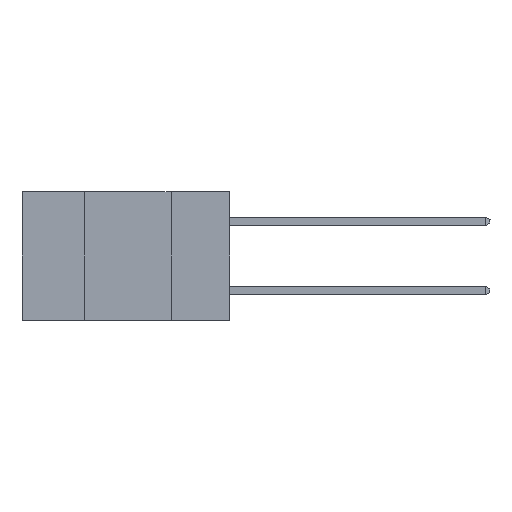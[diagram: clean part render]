
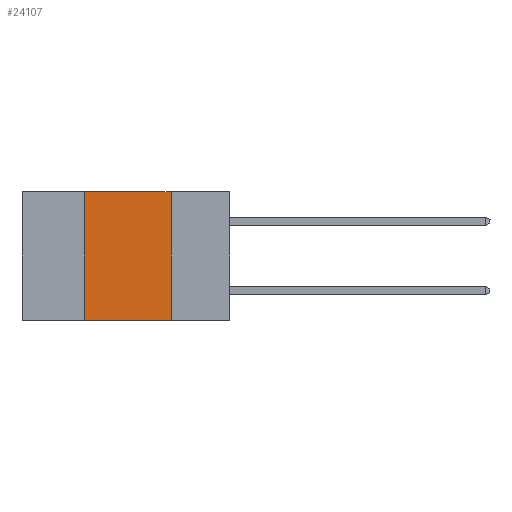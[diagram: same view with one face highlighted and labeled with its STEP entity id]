
A CAD part, left-side view. The second image highlights one B-rep face of the part: STEP entity #24107.
In plain terms, the highlighted planar face has unit normal (-1, 0, 0).
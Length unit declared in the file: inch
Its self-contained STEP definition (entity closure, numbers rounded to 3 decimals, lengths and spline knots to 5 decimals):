
#48 = ORIENTED_EDGE ( 'NONE', *, *, #21005, .F. ) ;
#402 = ORIENTED_EDGE ( 'NONE', *, *, #11952, .T. ) ;
#648 = VECTOR ( 'NONE', #15924, 39.37008 ) ;
#2300 = AXIS2_PLACEMENT_3D ( 'NONE', #16759, #10589, #20846 ) ;
#3152 = EDGE_LOOP ( 'NONE', ( #10377, #48, #4232, #402 ) ) ;
#3196 = CARTESIAN_POINT ( 'NONE',  ( 0., 0.17, 0. ) ) ;
#4232 = ORIENTED_EDGE ( 'NONE', *, *, #11881, .F. ) ;
#4392 = CARTESIAN_POINT ( 'NONE',  ( 0., 0.42, 0. ) ) ;
#4563 = VECTOR ( 'NONE', #9537, 39.37008 ) ;
#6471 = LINE ( 'NONE', #3196, #648 ) ;
#8811 = VECTOR ( 'NONE', #22418, 39.37008 ) ;
#9537 = DIRECTION ( 'NONE',  ( 0., -1., 0. ) ) ;
#9734 = VECTOR ( 'NONE', #11134, 39.37008 ) ;
#10377 = ORIENTED_EDGE ( 'NONE', *, *, #17803, .F. ) ;
#10589 = DIRECTION ( 'NONE',  ( 1., 0., 0. ) ) ;
#11052 = CARTESIAN_POINT ( 'NONE',  ( 0., 0.42, 0. ) ) ;
#11084 = LINE ( 'NONE', #11052, #9734 ) ;
#11134 = DIRECTION ( 'NONE',  ( 0., 0., 1. ) ) ;
#11881 = EDGE_CURVE ( 'NONE', #20860, #12257, #11084, .T. ) ;
#11952 = EDGE_CURVE ( 'NONE', #20860, #13655, #16928, .T. ) ;
#12257 = VERTEX_POINT ( 'NONE', #4392 ) ;
#13184 = CARTESIAN_POINT ( 'NONE',  ( 0., 0.17, -0.37 ) ) ;
#13655 = VERTEX_POINT ( 'NONE', #13184 ) ;
#15924 = DIRECTION ( 'NONE',  ( 0., 0., -1. ) ) ;
#16759 = CARTESIAN_POINT ( 'NONE',  ( 0., 0.6, 0. ) ) ;
#16928 = LINE ( 'NONE', #21991, #4563 ) ;
#17803 = EDGE_CURVE ( 'NONE', #22155, #13655, #6471, .T. ) ;
#19588 = LINE ( 'NONE', #24414, #8811 ) ;
#20658 = PLANE ( 'NONE',  #2300 ) ;
#20846 = DIRECTION ( 'NONE',  ( 0., 0., -1. ) ) ;
#20860 = VERTEX_POINT ( 'NONE', #21879 ) ;
#21005 = EDGE_CURVE ( 'NONE', #12257, #22155, #19588, .T. ) ;
#21879 = CARTESIAN_POINT ( 'NONE',  ( 0., 0.42, -0.37 ) ) ;
#21991 = CARTESIAN_POINT ( 'NONE',  ( 0., 0.6, -0.37 ) ) ;
#22155 = VERTEX_POINT ( 'NONE', #22356 ) ;
#22356 = CARTESIAN_POINT ( 'NONE',  ( 0., 0.17, 0. ) ) ;
#22418 = DIRECTION ( 'NONE',  ( 0., -1., 0. ) ) ;
#24107 = ADVANCED_FACE ( 'NONE', ( #25928 ), #20658, .F. ) ;
#24414 = CARTESIAN_POINT ( 'NONE',  ( 0., 0.6, 0. ) ) ;
#25928 = FACE_OUTER_BOUND ( 'NONE', #3152, .T. ) ;
